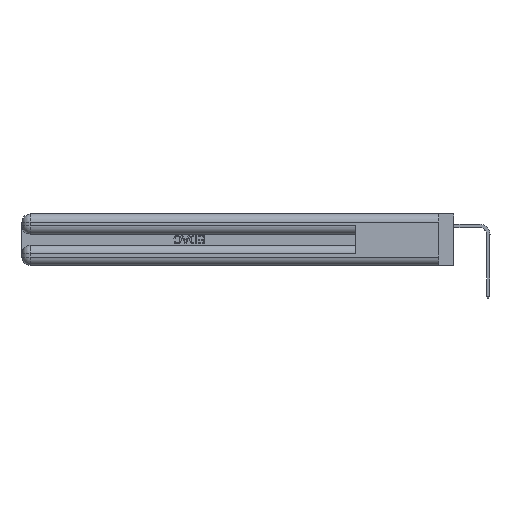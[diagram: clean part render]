
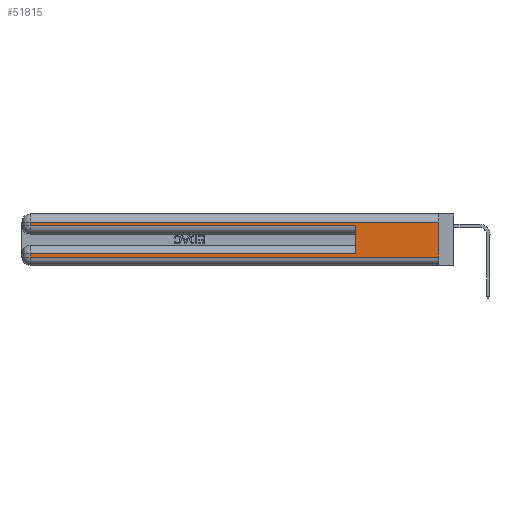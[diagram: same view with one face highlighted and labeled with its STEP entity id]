
A CAD part, left-side view. The second image highlights one B-rep face of the part: STEP entity #51815.
In plain terms, the highlighted planar face has unit normal (-1, 0, 0).
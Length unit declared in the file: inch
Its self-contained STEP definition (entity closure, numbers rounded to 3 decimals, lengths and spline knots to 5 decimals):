
#568 = LINE ( 'NONE', #36491, #54284 ) ;
#735 = CARTESIAN_POINT ( 'NONE',  ( 0., 0.6, 0.145 ) ) ;
#926 = DIRECTION ( 'NONE',  ( 0., 0., 1. ) ) ;
#1797 = EDGE_CURVE ( 'NONE', #45030, #52925, #5746, .T. ) ;
#1920 = LINE ( 'NONE', #23460, #23145 ) ;
#4388 = VECTOR ( 'NONE', #48044, 39.37008 ) ;
#5746 = LINE ( 'NONE', #26740, #4388 ) ;
#6205 = CARTESIAN_POINT ( 'NONE',  ( 0., 2.94, 0.06 ) ) ;
#6858 = VERTEX_POINT ( 'NONE', #37043 ) ;
#6873 = CARTESIAN_POINT ( 'NONE',  ( 0., 2.94, 0.085 ) ) ;
#7112 = VERTEX_POINT ( 'NONE', #51425 ) ;
#8476 = AXIS2_PLACEMENT_3D ( 'NONE', #20182, #49829, #24444 ) ;
#8530 = LINE ( 'NONE', #30363, #29754 ) ;
#11499 = VECTOR ( 'NONE', #22149, 39.37008 ) ;
#11681 = PLANE ( 'NONE',  #8476 ) ;
#12120 = EDGE_CURVE ( 'NONE', #7112, #21191, #46630, .T. ) ;
#14339 = CARTESIAN_POINT ( 'NONE',  ( 0., 0.6, 0.085 ) ) ;
#14842 = EDGE_CURVE ( 'NONE', #22919, #6858, #8530, .T. ) ;
#14983 = CARTESIAN_POINT ( 'NONE',  ( 0., 2.94, 0.31 ) ) ;
#17517 = VECTOR ( 'NONE', #22614, 39.37008 ) ;
#17920 = CARTESIAN_POINT ( 'NONE',  ( 0., 0., 0.31 ) ) ;
#19403 = DIRECTION ( 'NONE',  ( 0., 0., -1. ) ) ;
#20165 = CARTESIAN_POINT ( 'NONE',  ( 0., 0., 0.085 ) ) ;
#20182 = CARTESIAN_POINT ( 'NONE',  ( 0., 0., 0.37 ) ) ;
#20642 = EDGE_CURVE ( 'NONE', #37867, #45030, #50096, .T. ) ;
#21191 = VERTEX_POINT ( 'NONE', #14983 ) ;
#22101 = EDGE_CURVE ( 'NONE', #52925, #31541, #30135, .T. ) ;
#22149 = DIRECTION ( 'NONE',  ( 0., 1., 0. ) ) ;
#22614 = DIRECTION ( 'NONE',  ( 0., -1., 0. ) ) ;
#22785 = ORIENTED_EDGE ( 'NONE', *, *, #48571, .T. ) ;
#22919 = VERTEX_POINT ( 'NONE', #32536 ) ;
#23100 = ORIENTED_EDGE ( 'NONE', *, *, #14842, .T. ) ;
#23145 = VECTOR ( 'NONE', #27749, 39.37008 ) ;
#23460 = CARTESIAN_POINT ( 'NONE',  ( 0., 2.94, 0.37 ) ) ;
#23891 = ORIENTED_EDGE ( 'NONE', *, *, #47858, .F. ) ;
#24444 = DIRECTION ( 'NONE',  ( 0., 0., -1. ) ) ;
#26740 = CARTESIAN_POINT ( 'NONE',  ( 0., 2.94, 0.37 ) ) ;
#27749 = DIRECTION ( 'NONE',  ( 0., 0., -1. ) ) ;
#28075 = ORIENTED_EDGE ( 'NONE', *, *, #12120, .T. ) ;
#29754 = VECTOR ( 'NONE', #34593, 39.37008 ) ;
#30135 = LINE ( 'NONE', #52266, #17517 ) ;
#30254 = EDGE_CURVE ( 'NONE', #7112, #31541, #568, .T. ) ;
#30363 = CARTESIAN_POINT ( 'NONE',  ( 0., 0., 0.285 ) ) ;
#31541 = VERTEX_POINT ( 'NONE', #44020 ) ;
#31910 = ORIENTED_EDGE ( 'NONE', *, *, #20642, .T. ) ;
#32536 = CARTESIAN_POINT ( 'NONE',  ( 0., 2.94, 0.285 ) ) ;
#34593 = DIRECTION ( 'NONE',  ( 0., -1., 0. ) ) ;
#34726 = FACE_OUTER_BOUND ( 'NONE', #47031, .T. ) ;
#36491 = CARTESIAN_POINT ( 'NONE',  ( 0., 0., 0.37 ) ) ;
#36895 = DIRECTION ( 'NONE',  ( 0., 1., 0. ) ) ;
#37043 = CARTESIAN_POINT ( 'NONE',  ( 0., 0.6, 0.285 ) ) ;
#37867 = VERTEX_POINT ( 'NONE', #14339 ) ;
#39220 = VECTOR ( 'NONE', #926, 39.37008 ) ;
#42526 = ORIENTED_EDGE ( 'NONE', *, *, #22101, .T. ) ;
#44020 = CARTESIAN_POINT ( 'NONE',  ( 0., 0., 0.06 ) ) ;
#45030 = VERTEX_POINT ( 'NONE', #6873 ) ;
#46630 = LINE ( 'NONE', #17920, #11499 ) ;
#47031 = EDGE_LOOP ( 'NONE', ( #51214, #28075, #22785, #23100, #23891, #31910, #48440, #42526 ) ) ;
#47432 = VECTOR ( 'NONE', #36895, 39.37008 ) ;
#47858 = EDGE_CURVE ( 'NONE', #37867, #6858, #51758, .T. ) ;
#48044 = DIRECTION ( 'NONE',  ( 0., 0., -1. ) ) ;
#48440 = ORIENTED_EDGE ( 'NONE', *, *, #1797, .T. ) ;
#48571 = EDGE_CURVE ( 'NONE', #21191, #22919, #1920, .T. ) ;
#49829 = DIRECTION ( 'NONE',  ( 1., 0., 0. ) ) ;
#50096 = LINE ( 'NONE', #20165, #47432 ) ;
#51214 = ORIENTED_EDGE ( 'NONE', *, *, #30254, .F. ) ;
#51425 = CARTESIAN_POINT ( 'NONE',  ( 0., 0., 0.31 ) ) ;
#51758 = LINE ( 'NONE', #735, #39220 ) ;
#51815 = ADVANCED_FACE ( 'NONE', ( #34726 ), #11681, .F. ) ;
#52266 = CARTESIAN_POINT ( 'NONE',  ( 0., 0., 0.06 ) ) ;
#52925 = VERTEX_POINT ( 'NONE', #6205 ) ;
#54284 = VECTOR ( 'NONE', #19403, 39.37008 ) ;
